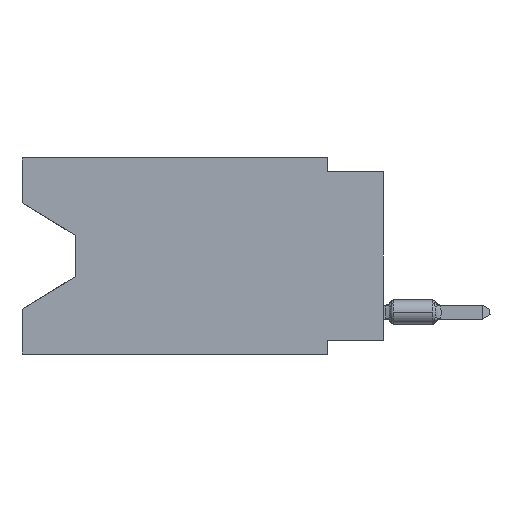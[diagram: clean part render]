
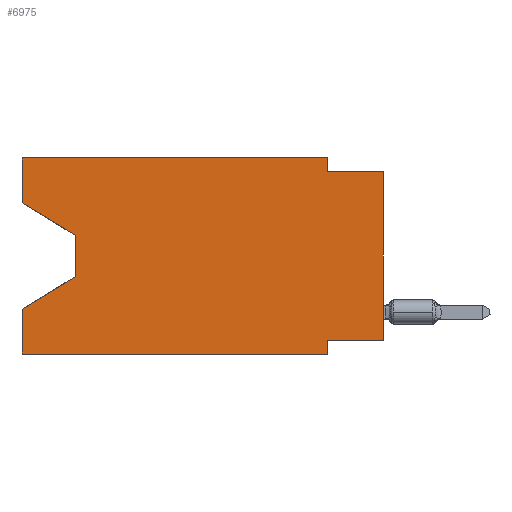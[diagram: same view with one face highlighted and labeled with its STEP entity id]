
A CAD part, left-side view. The second image highlights one B-rep face of the part: STEP entity #6975.
In plain terms, the highlighted planar face has unit normal (-1, 0, 0).
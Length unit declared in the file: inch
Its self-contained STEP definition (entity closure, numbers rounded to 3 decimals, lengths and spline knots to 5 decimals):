
#292 = VERTEX_POINT ( 'NONE', #17073 ) ;
#299 = DIRECTION ( 'NONE',  ( 0., -1., 0. ) ) ;
#878 = VECTOR ( 'NONE', #8012, 39.37008 ) ;
#1101 = DIRECTION ( 'NONE',  ( 0., -1., 0. ) ) ;
#1163 = ORIENTED_EDGE ( 'NONE', *, *, #6809, .T. ) ;
#1289 = CARTESIAN_POINT ( 'NONE',  ( 0., 0., -0.325 ) ) ;
#1385 = AXIS2_PLACEMENT_3D ( 'NONE', #10116, #20020, #15078 ) ;
#1660 = CARTESIAN_POINT ( 'NONE',  ( 0., 0., 0. ) ) ;
#2100 = LINE ( 'NONE', #11769, #19779 ) ;
#2277 = VERTEX_POINT ( 'NONE', #15622 ) ;
#2354 = EDGE_CURVE ( 'NONE', #14004, #6635, #10892, .T. ) ;
#2874 = ORIENTED_EDGE ( 'NONE', *, *, #2354, .T. ) ;
#2940 = EDGE_CURVE ( 'NONE', #10329, #9728, #10169, .T. ) ;
#3001 = CARTESIAN_POINT ( 'NONE',  ( 0., 0.1, -0.35 ) ) ;
#3105 = CARTESIAN_POINT ( 'NONE',  ( 0., 0.55, -0.138 ) ) ;
#3155 = VECTOR ( 'NONE', #299, 39.37008 ) ;
#3268 = CARTESIAN_POINT ( 'NONE',  ( 0., 0.1, 0. ) ) ;
#3509 = EDGE_CURVE ( 'NONE', #2277, #292, #6209, .T. ) ;
#3520 = EDGE_CURVE ( 'NONE', #292, #3796, #17731, .T. ) ;
#3796 = VERTEX_POINT ( 'NONE', #5548 ) ;
#3799 = ORIENTED_EDGE ( 'NONE', *, *, #4216, .T. ) ;
#4216 = EDGE_CURVE ( 'NONE', #17437, #3796, #13776, .T. ) ;
#4364 = LINE ( 'NONE', #21011, #4382 ) ;
#4382 = VECTOR ( 'NONE', #12413, 39.37008 ) ;
#4608 = CARTESIAN_POINT ( 'NONE',  ( 0., 0., -0.025 ) ) ;
#4684 = ORIENTED_EDGE ( 'NONE', *, *, #16474, .F. ) ;
#4828 = DIRECTION ( 'NONE',  ( 0., 1., 0. ) ) ;
#5065 = ORIENTED_EDGE ( 'NONE', *, *, #2940, .F. ) ;
#5392 = EDGE_CURVE ( 'NONE', #17437, #12939, #2100, .T. ) ;
#5548 = CARTESIAN_POINT ( 'NONE',  ( 0., 0.1, -0.35 ) ) ;
#6209 = LINE ( 'NONE', #1289, #6394 ) ;
#6394 = VECTOR ( 'NONE', #4828, 39.37008 ) ;
#6486 = LINE ( 'NONE', #3268, #6852 ) ;
#6635 = VERTEX_POINT ( 'NONE', #19067 ) ;
#6740 = ORIENTED_EDGE ( 'NONE', *, *, #5392, .F. ) ;
#6809 = EDGE_CURVE ( 'NONE', #2277, #9728, #14765, .T. ) ;
#6852 = VECTOR ( 'NONE', #13051, 39.37008 ) ;
#6975 = ADVANCED_FACE ( 'NONE', ( #10334 ), #13466, .F. ) ;
#7384 = EDGE_CURVE ( 'NONE', #8250, #10329, #6486, .T. ) ;
#8012 = DIRECTION ( 'NONE',  ( 0., 0., 1. ) ) ;
#8133 = ORIENTED_EDGE ( 'NONE', *, *, #3509, .F. ) ;
#8250 = VERTEX_POINT ( 'NONE', #18066 ) ;
#8565 = CARTESIAN_POINT ( 'NONE',  ( 0., 0., -0.025 ) ) ;
#8844 = EDGE_CURVE ( 'NONE', #16321, #8250, #15319, .T. ) ;
#9246 = VECTOR ( 'NONE', #14452, 39.37008 ) ;
#9483 = CARTESIAN_POINT ( 'NONE',  ( 0., 0.55, -0.138 ) ) ;
#9728 = VERTEX_POINT ( 'NONE', #4608 ) ;
#9917 = VECTOR ( 'NONE', #20889, 39.37008 ) ;
#10116 = CARTESIAN_POINT ( 'NONE',  ( 0., 0.645, 0. ) ) ;
#10169 = LINE ( 'NONE', #8565, #20234 ) ;
#10329 = VERTEX_POINT ( 'NONE', #19619 ) ;
#10334 = FACE_OUTER_BOUND ( 'NONE', #10536, .T. ) ;
#10522 = EDGE_CURVE ( 'NONE', #13433, #14004, #12178, .T. ) ;
#10536 = EDGE_LOOP ( 'NONE', ( #12860, #2874, #20969, #6740, #3799, #13473, #8133, #1163, #5065, #14335, #19500, #4684 ) ) ;
#10892 = LINE ( 'NONE', #9483, #9917 ) ;
#10993 = CARTESIAN_POINT ( 'NONE',  ( 0., 0.645, -0.08025 ) ) ;
#11769 = CARTESIAN_POINT ( 'NONE',  ( 0., 0.645, 0. ) ) ;
#12178 = LINE ( 'NONE', #10993, #20632 ) ;
#12413 = DIRECTION ( 'NONE',  ( 0., 0.855, -0.519 ) ) ;
#12773 = DIRECTION ( 'NONE',  ( 0., 0., -1. ) ) ;
#12860 = ORIENTED_EDGE ( 'NONE', *, *, #10522, .T. ) ;
#12939 = VERTEX_POINT ( 'NONE', #15197 ) ;
#12971 = CARTESIAN_POINT ( 'NONE',  ( 0., 0.645, 0. ) ) ;
#13051 = DIRECTION ( 'NONE',  ( 0., 0., -1. ) ) ;
#13433 = VERTEX_POINT ( 'NONE', #20322 ) ;
#13466 = PLANE ( 'NONE',  #1385 ) ;
#13473 = ORIENTED_EDGE ( 'NONE', *, *, #3520, .F. ) ;
#13576 = VECTOR ( 'NONE', #1101, 39.37008 ) ;
#13776 = LINE ( 'NONE', #17546, #13576 ) ;
#14004 = VERTEX_POINT ( 'NONE', #3105 ) ;
#14335 = ORIENTED_EDGE ( 'NONE', *, *, #7384, .F. ) ;
#14452 = DIRECTION ( 'NONE',  ( 0., 0., 1. ) ) ;
#14639 = VECTOR ( 'NONE', #12773, 39.37008 ) ;
#14765 = LINE ( 'NONE', #1660, #9246 ) ;
#15078 = DIRECTION ( 'NONE',  ( 0., 0., -1. ) ) ;
#15126 = DIRECTION ( 'NONE',  ( 0., -1., 0. ) ) ;
#15137 = CARTESIAN_POINT ( 'NONE',  ( 0., 0.645, -0.35 ) ) ;
#15197 = CARTESIAN_POINT ( 'NONE',  ( 0., 0.645, -0.26975 ) ) ;
#15319 = LINE ( 'NONE', #18348, #3155 ) ;
#15622 = CARTESIAN_POINT ( 'NONE',  ( 0., 0., -0.325 ) ) ;
#16321 = VERTEX_POINT ( 'NONE', #17065 ) ;
#16474 = EDGE_CURVE ( 'NONE', #13433, #16321, #16508, .T. ) ;
#16508 = LINE ( 'NONE', #12971, #878 ) ;
#17065 = CARTESIAN_POINT ( 'NONE',  ( 0., 0.645, 0. ) ) ;
#17073 = CARTESIAN_POINT ( 'NONE',  ( 0., 0.1, -0.325 ) ) ;
#17437 = VERTEX_POINT ( 'NONE', #15137 ) ;
#17546 = CARTESIAN_POINT ( 'NONE',  ( 0., 0.645, -0.35 ) ) ;
#17562 = DIRECTION ( 'NONE',  ( 0., -0.855, -0.519 ) ) ;
#17731 = LINE ( 'NONE', #3001, #14639 ) ;
#18066 = CARTESIAN_POINT ( 'NONE',  ( 0., 0.1, 0. ) ) ;
#18348 = CARTESIAN_POINT ( 'NONE',  ( 0., 0.645, 0. ) ) ;
#19067 = CARTESIAN_POINT ( 'NONE',  ( 0., 0.55, -0.212 ) ) ;
#19500 = ORIENTED_EDGE ( 'NONE', *, *, #8844, .F. ) ;
#19619 = CARTESIAN_POINT ( 'NONE',  ( 0., 0.1, -0.025 ) ) ;
#19779 = VECTOR ( 'NONE', #20039, 39.37008 ) ;
#20020 = DIRECTION ( 'NONE',  ( 1., 0., 0. ) ) ;
#20039 = DIRECTION ( 'NONE',  ( 0., 0., 1. ) ) ;
#20128 = EDGE_CURVE ( 'NONE', #6635, #12939, #4364, .T. ) ;
#20234 = VECTOR ( 'NONE', #15126, 39.37008 ) ;
#20322 = CARTESIAN_POINT ( 'NONE',  ( 0., 0.645, -0.08025 ) ) ;
#20632 = VECTOR ( 'NONE', #17562, 39.37008 ) ;
#20889 = DIRECTION ( 'NONE',  ( 0., 0., -1. ) ) ;
#20969 = ORIENTED_EDGE ( 'NONE', *, *, #20128, .T. ) ;
#21011 = CARTESIAN_POINT ( 'NONE',  ( 0., 0.55, -0.212 ) ) ;
